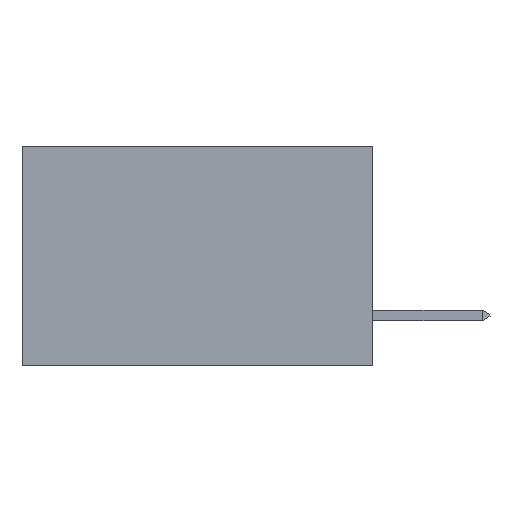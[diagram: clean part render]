
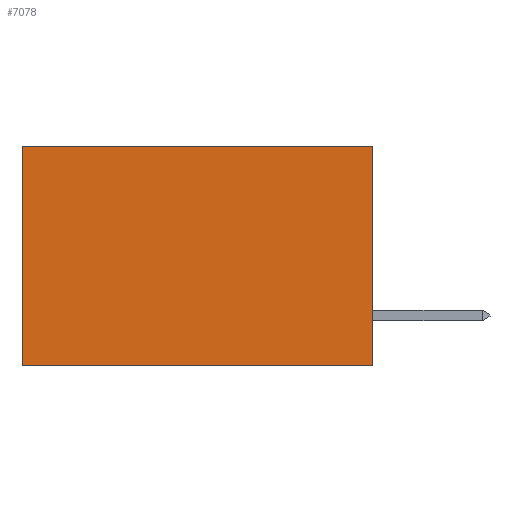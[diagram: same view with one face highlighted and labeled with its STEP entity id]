
A CAD part, left-side view. The second image highlights one B-rep face of the part: STEP entity #7078.
In plain terms, the highlighted planar face has unit normal (-1, 0, 0).
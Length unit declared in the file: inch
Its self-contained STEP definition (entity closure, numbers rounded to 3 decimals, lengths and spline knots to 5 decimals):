
#217 = DIRECTION ( 'NONE',  ( 0., 0., -1. ) ) ;
#383 = ORIENTED_EDGE ( 'NONE', *, *, #9908, .T. ) ;
#481 = EDGE_CURVE ( 'NONE', #6675, #4863, #10024, .T. ) ;
#506 = FACE_OUTER_BOUND ( 'NONE', #3242, .T. ) ;
#1391 = DIRECTION ( 'NONE',  ( 0., 1., 0. ) ) ;
#1472 = ORIENTED_EDGE ( 'NONE', *, *, #481, .F. ) ;
#1652 = EDGE_CURVE ( 'NONE', #9375, #7954, #5872, .T. ) ;
#1693 = VECTOR ( 'NONE', #4573, 39.37008 ) ;
#2769 = AXIS2_PLACEMENT_3D ( 'NONE', #3368, #3344, #3316 ) ;
#3242 = EDGE_LOOP ( 'NONE', ( #383, #1472, #4991, #7260 ) ) ;
#3316 = DIRECTION ( 'NONE',  ( 0., 0., -1. ) ) ;
#3344 = DIRECTION ( 'NONE',  ( 1., 0., 0. ) ) ;
#3368 = CARTESIAN_POINT ( 'NONE',  ( 0.277, 0., -0.37 ) ) ;
#3384 = PLANE ( 'NONE',  #2769 ) ;
#3424 = DIRECTION ( 'NONE',  ( 0., 0., -1. ) ) ;
#3469 = CARTESIAN_POINT ( 'NONE',  ( 0.277, 0., -0.37 ) ) ;
#4573 = DIRECTION ( 'NONE',  ( 0., 1., 0. ) ) ;
#4863 = VERTEX_POINT ( 'NONE', #8691 ) ;
#4991 = ORIENTED_EDGE ( 'NONE', *, *, #8078, .F. ) ;
#5872 = LINE ( 'NONE', #10196, #9882 ) ;
#6085 = CARTESIAN_POINT ( 'NONE',  ( 0.277, 0., -0.37 ) ) ;
#6675 = VERTEX_POINT ( 'NONE', #6085 ) ;
#6703 = CARTESIAN_POINT ( 'NONE',  ( 0.277, 0.59, 0. ) ) ;
#6833 = CARTESIAN_POINT ( 'NONE',  ( 0.277, 0., 0. ) ) ;
#7078 = ADVANCED_FACE ( 'NONE', ( #506 ), #3384, .F. ) ;
#7260 = ORIENTED_EDGE ( 'NONE', *, *, #1652, .T. ) ;
#7602 = CARTESIAN_POINT ( 'NONE',  ( 0.277, 0., -0.37 ) ) ;
#7954 = VERTEX_POINT ( 'NONE', #6703 ) ;
#8078 = EDGE_CURVE ( 'NONE', #9375, #6675, #9064, .T. ) ;
#8239 = VECTOR ( 'NONE', #217, 39.37008 ) ;
#8691 = CARTESIAN_POINT ( 'NONE',  ( 0.277, 0.59, -0.37 ) ) ;
#9064 = LINE ( 'NONE', #3469, #10293 ) ;
#9375 = VERTEX_POINT ( 'NONE', #6833 ) ;
#9759 = CARTESIAN_POINT ( 'NONE',  ( 0.277, 0.59, -0.37 ) ) ;
#9882 = VECTOR ( 'NONE', #1391, 39.37008 ) ;
#9908 = EDGE_CURVE ( 'NONE', #7954, #4863, #10274, .T. ) ;
#10024 = LINE ( 'NONE', #7602, #1693 ) ;
#10196 = CARTESIAN_POINT ( 'NONE',  ( 0.277, 0., 0. ) ) ;
#10274 = LINE ( 'NONE', #9759, #8239 ) ;
#10293 = VECTOR ( 'NONE', #3424, 39.37008 ) ;
